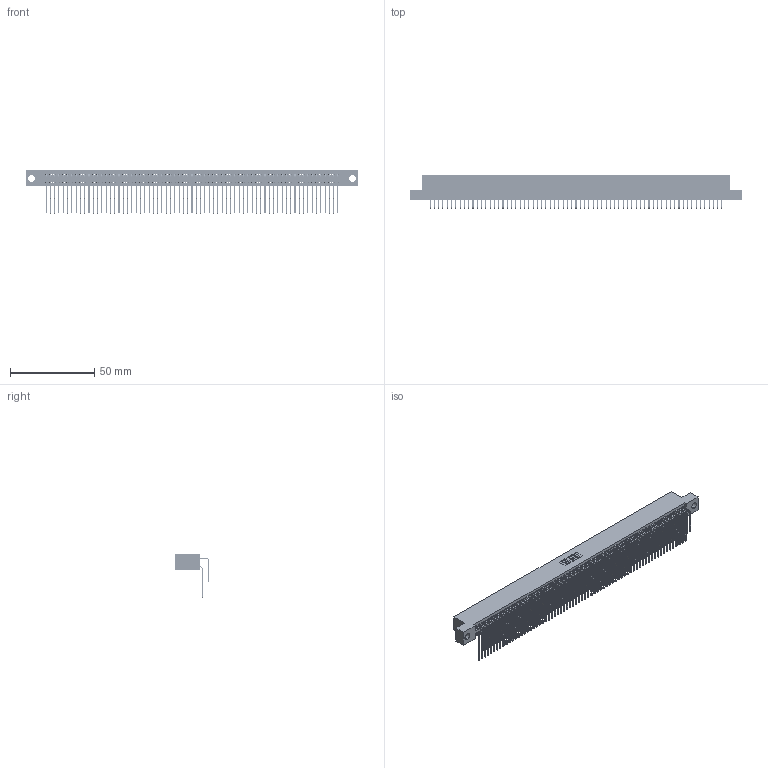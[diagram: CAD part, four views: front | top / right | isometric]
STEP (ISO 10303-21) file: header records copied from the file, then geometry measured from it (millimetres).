
FILE_DESCRIPTION (( 'STEP AP203' ), '1' );
FILE_NAME ('395-138-559-204.STEP', '2021-06-18T03:59:37', ( '' ), ( '' ), 'SwSTEP 2.0', 'SolidWorks 2020', '' );
FILE_SCHEMA (( 'CONFIG_CONTROL_DESIGN' ));
Length unit declared in the file: inch
Products named in the file (4): 345-292-001_558 559 Tail - 1; 345 Part_Flush Mounting Lugs - 0.156 Dia-TI; 345-292-001_559 Tail - 2; 395-138-559-204
Assembly tree (139 placements, depth 2):
  395-138-559-204
    345 Part_Flush Mounting Lugs - 0.156 Dia-TI
    345-292-001_558 559 Tail - 1  x69
    345-292-001_559 Tail - 2  x69
Bounding box: 196.47 x 20.56 x 25.53 mm (x, y, z)
Volume: 20026 mm3; surface area: 33719.7 mm2
Topology: 139 solids, 139 shells, 7316 faces, 21767 edges, 14326 vertices
Faces by surface type: plane 4924, cylinder 2392
Entity records: 52575 total; most frequent: CARTESIAN_POINT 8837, ORIENTED_EDGE 8718, DIRECTION 7731, EDGE_CURVE 4359, VECTOR 3911, LINE 3911, VERTEX_POINT 2902, AXIS2_PLACEMENT_3D 1910
